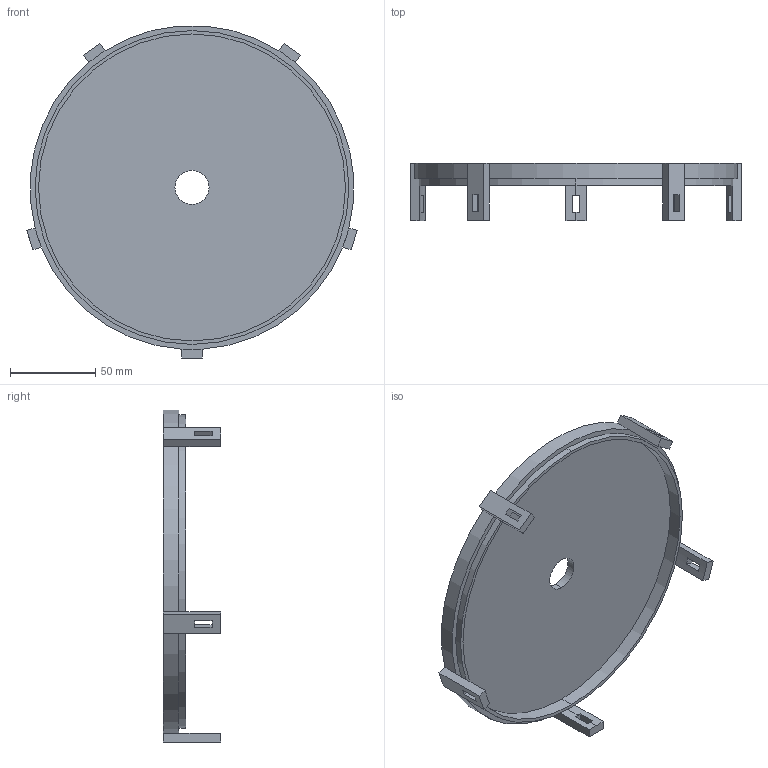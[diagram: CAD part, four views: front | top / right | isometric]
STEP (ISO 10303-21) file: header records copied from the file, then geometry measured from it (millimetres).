
FILE_DESCRIPTION (( 'STEP AP203' ), '1' );
FILE_NAME ('rear.STEP', '2013-09-09T02:44:00', ( '' ), ( '' ), 'SwSTEP 2.0', 'SolidWorks 2013', '' );
FILE_SCHEMA (( 'CONFIG_CONTROL_DESIGN' ));
Length unit declared in the file: millimetre
Products named in the file (1): rear
Bounding box: 193.85 x 33.46 x 194.69 mm (x, y, z)
Volume: 165338.3 mm3; surface area: 74118.6 mm2
Topology: 1 solids, 1 shells, 69 faces, 185 edges, 120 vertices
Faces by surface type: plane 50, cylinder 19
Entity records: 2250 total; most frequent: DIRECTION 375, CARTESIAN_POINT 375, ORIENTED_EDGE 370, EDGE_CURVE 185, LINE 135, VECTOR 135, VERTEX_POINT 120, AXIS2_PLACEMENT_3D 120
